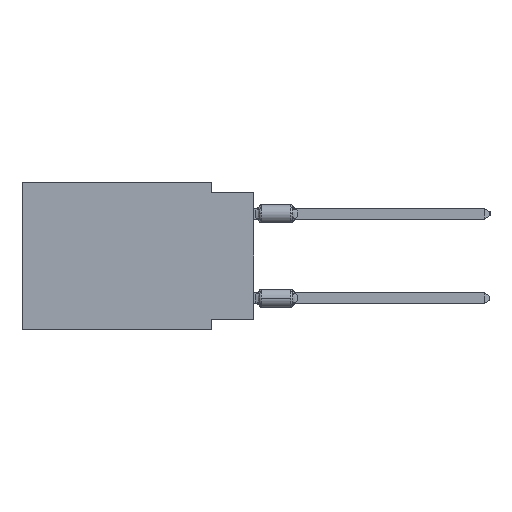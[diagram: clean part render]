
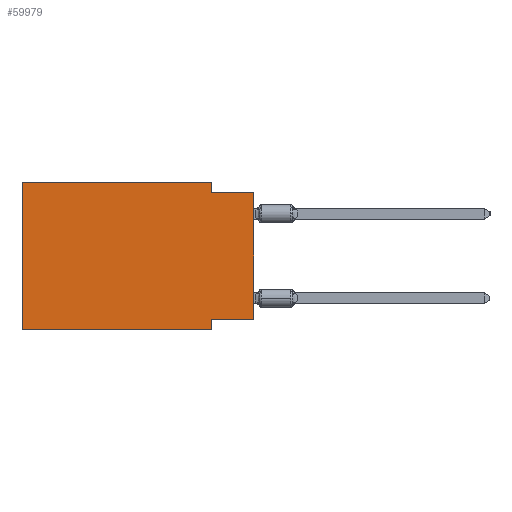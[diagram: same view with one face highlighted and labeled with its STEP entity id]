
A CAD part, left-side view. The second image highlights one B-rep face of the part: STEP entity #59979.
In plain terms, the highlighted planar face has unit normal (-1, 0, 0).
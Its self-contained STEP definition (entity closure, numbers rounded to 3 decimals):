
#253 = EDGE_CURVE ( 'NONE', #12944, #63262, #4984, .T. ) ;
#963 = VERTEX_POINT ( 'NONE', #55960 ) ;
#1489 = CARTESIAN_POINT ( 'NONE',  ( 0., 13.97, -8.89 ) ) ;
#2234 = LINE ( 'NONE', #42354, #35245 ) ;
#3520 = CARTESIAN_POINT ( 'NONE',  ( 0., 0., -8.255 ) ) ;
#3598 = FACE_OUTER_BOUND ( 'NONE', #16991, .T. ) ;
#4984 = LINE ( 'NONE', #54911, #34308 ) ;
#4998 = CARTESIAN_POINT ( 'NONE',  ( 0., 2.54, 0. ) ) ;
#5194 = DIRECTION ( 'NONE',  ( 0., 0., -1. ) ) ;
#5838 = CARTESIAN_POINT ( 'NONE',  ( 0., 2.54, 0. ) ) ;
#6184 = CARTESIAN_POINT ( 'NONE',  ( 0., 2.54, -8.255 ) ) ;
#6979 = CARTESIAN_POINT ( 'NONE',  ( 0., 0., -0.635 ) ) ;
#8405 = ORIENTED_EDGE ( 'NONE', *, *, #10217, .F. ) ;
#8809 = DIRECTION ( 'NONE',  ( 1., 0., 0. ) ) ;
#9487 = EDGE_CURVE ( 'NONE', #14309, #963, #38615, .T. ) ;
#9879 = DIRECTION ( 'NONE',  ( 0., -1., 0. ) ) ;
#10217 = EDGE_CURVE ( 'NONE', #60307, #14309, #40857, .T. ) ;
#12944 = VERTEX_POINT ( 'NONE', #24285 ) ;
#14309 = VERTEX_POINT ( 'NONE', #6184 ) ;
#16991 = EDGE_LOOP ( 'NONE', ( #45264, #57140, #27226, #26829, #59117, #50187, #62857, #8405 ) ) ;
#18598 = DIRECTION ( 'NONE',  ( 0., 0., -1. ) ) ;
#18680 = LINE ( 'NONE', #58474, #21509 ) ;
#19779 = EDGE_CURVE ( 'NONE', #41296, #12944, #2234, .T. ) ;
#21509 = VECTOR ( 'NONE', #42828, 1000. ) ;
#21942 = VERTEX_POINT ( 'NONE', #6979 ) ;
#22683 = CARTESIAN_POINT ( 'NONE',  ( 0., 2.54, -8.89 ) ) ;
#23475 = VECTOR ( 'NONE', #51391, 1000. ) ;
#24285 = CARTESIAN_POINT ( 'NONE',  ( 0., 13.97, 0. ) ) ;
#26829 = ORIENTED_EDGE ( 'NONE', *, *, #253, .F. ) ;
#27226 = ORIENTED_EDGE ( 'NONE', *, *, #29779, .F. ) ;
#27722 = VECTOR ( 'NONE', #57254, 1000. ) ;
#29779 = EDGE_CURVE ( 'NONE', #63262, #59153, #59667, .T. ) ;
#34308 = VECTOR ( 'NONE', #9879, 1000. ) ;
#34797 = VECTOR ( 'NONE', #39287, 1000. ) ;
#35245 = VECTOR ( 'NONE', #41376, 1000. ) ;
#35972 = DIRECTION ( 'NONE',  ( 0., 1., 0. ) ) ;
#38486 = CARTESIAN_POINT ( 'NONE',  ( 0., 13.97, 0. ) ) ;
#38615 = LINE ( 'NONE', #22683, #27722 ) ;
#38804 = PLANE ( 'NONE',  #49247 ) ;
#39287 = DIRECTION ( 'NONE',  ( 0., -1., 0. ) ) ;
#40857 = LINE ( 'NONE', #60766, #53792 ) ;
#41296 = VERTEX_POINT ( 'NONE', #56187 ) ;
#41376 = DIRECTION ( 'NONE',  ( 0., 0., 1. ) ) ;
#42354 = CARTESIAN_POINT ( 'NONE',  ( 0., 13.97, 0. ) ) ;
#42828 = DIRECTION ( 'NONE',  ( 0., 0., 1. ) ) ;
#44503 = CARTESIAN_POINT ( 'NONE',  ( 0., 0., -0.635 ) ) ;
#45264 = ORIENTED_EDGE ( 'NONE', *, *, #47664, .T. ) ;
#47306 = EDGE_CURVE ( 'NONE', #59153, #21942, #59190, .T. ) ;
#47664 = EDGE_CURVE ( 'NONE', #60307, #21942, #18680, .T. ) ;
#49247 = AXIS2_PLACEMENT_3D ( 'NONE', #38486, #8809, #18598 ) ;
#50187 = ORIENTED_EDGE ( 'NONE', *, *, #64242, .T. ) ;
#51391 = DIRECTION ( 'NONE',  ( 0., -1., 0. ) ) ;
#53792 = VECTOR ( 'NONE', #35972, 1000. ) ;
#54911 = CARTESIAN_POINT ( 'NONE',  ( 0., 13.97, 0. ) ) ;
#55960 = CARTESIAN_POINT ( 'NONE',  ( 0., 2.54, -8.89 ) ) ;
#56187 = CARTESIAN_POINT ( 'NONE',  ( 0., 13.97, -8.89 ) ) ;
#56621 = LINE ( 'NONE', #1489, #23475 ) ;
#57140 = ORIENTED_EDGE ( 'NONE', *, *, #47306, .F. ) ;
#57254 = DIRECTION ( 'NONE',  ( 0., 0., -1. ) ) ;
#57672 = CARTESIAN_POINT ( 'NONE',  ( 0., 2.54, -0.635 ) ) ;
#58474 = CARTESIAN_POINT ( 'NONE',  ( 0., 0., 0. ) ) ;
#58759 = VECTOR ( 'NONE', #5194, 1000. ) ;
#59117 = ORIENTED_EDGE ( 'NONE', *, *, #19779, .F. ) ;
#59153 = VERTEX_POINT ( 'NONE', #57672 ) ;
#59190 = LINE ( 'NONE', #44503, #34797 ) ;
#59667 = LINE ( 'NONE', #5838, #58759 ) ;
#59979 = ADVANCED_FACE ( 'NONE', ( #3598 ), #38804, .F. ) ;
#60307 = VERTEX_POINT ( 'NONE', #3520 ) ;
#60766 = CARTESIAN_POINT ( 'NONE',  ( 0., 0., -8.255 ) ) ;
#62857 = ORIENTED_EDGE ( 'NONE', *, *, #9487, .F. ) ;
#63262 = VERTEX_POINT ( 'NONE', #4998 ) ;
#64242 = EDGE_CURVE ( 'NONE', #41296, #963, #56621, .T. ) ;
